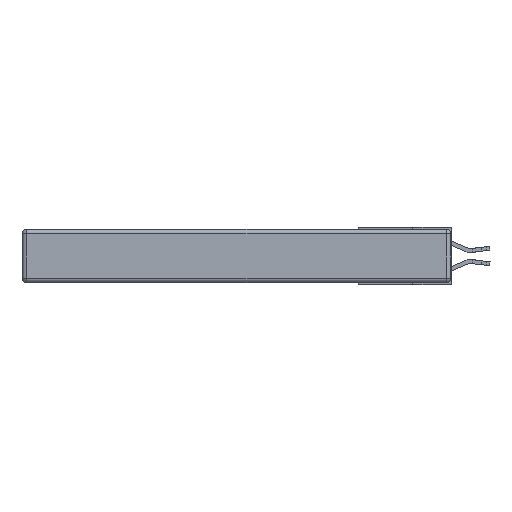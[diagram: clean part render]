
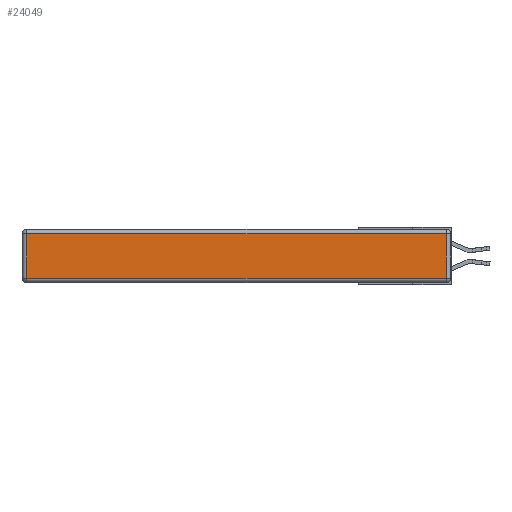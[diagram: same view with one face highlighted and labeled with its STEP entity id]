
A CAD part, left-side view. The second image highlights one B-rep face of the part: STEP entity #24049.
In plain terms, the highlighted planar face has unit normal (-1, 0, 0).
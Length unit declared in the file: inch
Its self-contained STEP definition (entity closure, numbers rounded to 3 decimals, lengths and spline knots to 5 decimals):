
#45 = LINE ( 'NONE', #12397, #9045 ) ;
#1283 = CARTESIAN_POINT ( 'NONE',  ( 0., 0.03, -0.313 ) ) ;
#1310 = DIRECTION ( 'NONE',  ( 0., 0., -1. ) ) ;
#3120 = DIRECTION ( 'NONE',  ( 0., -1., 0. ) ) ;
#3416 = EDGE_CURVE ( 'NONE', #7017, #4889, #10601, .T. ) ;
#4889 = VERTEX_POINT ( 'NONE', #5390 ) ;
#4909 = EDGE_CURVE ( 'NONE', #14106, #7017, #11949, .T. ) ;
#5390 = CARTESIAN_POINT ( 'NONE',  ( 0., 2.72, -0.03 ) ) ;
#5396 = EDGE_CURVE ( 'NONE', #4889, #11838, #45, .T. ) ;
#6542 = CARTESIAN_POINT ( 'NONE',  ( 0., 0., -0.313 ) ) ;
#6829 = CARTESIAN_POINT ( 'NONE',  ( 0., 0.03, -0.03 ) ) ;
#7017 = VERTEX_POINT ( 'NONE', #6829 ) ;
#7033 = CARTESIAN_POINT ( 'NONE',  ( 0., 0.03, -0.343 ) ) ;
#7079 = ORIENTED_EDGE ( 'NONE', *, *, #3416, .T. ) ;
#7637 = PLANE ( 'NONE',  #8991 ) ;
#8047 = ORIENTED_EDGE ( 'NONE', *, *, #17946, .T. ) ;
#8991 = AXIS2_PLACEMENT_3D ( 'NONE', #9500, #22446, #11336 ) ;
#9045 = VECTOR ( 'NONE', #1310, 39.37008 ) ;
#9436 = ORIENTED_EDGE ( 'NONE', *, *, #4909, .T. ) ;
#9500 = CARTESIAN_POINT ( 'NONE',  ( 0., 0., -0.343 ) ) ;
#10601 = LINE ( 'NONE', #21726, #21594 ) ;
#10744 = DIRECTION ( 'NONE',  ( 0., 0., 1. ) ) ;
#11041 = CARTESIAN_POINT ( 'NONE',  ( 0., 2.72, -0.313 ) ) ;
#11336 = DIRECTION ( 'NONE',  ( 0., 0., 1. ) ) ;
#11838 = VERTEX_POINT ( 'NONE', #11041 ) ;
#11949 = LINE ( 'NONE', #7033, #16877 ) ;
#12397 = CARTESIAN_POINT ( 'NONE',  ( 0., 2.72, -0.343 ) ) ;
#12641 = DIRECTION ( 'NONE',  ( 0., 1., 0. ) ) ;
#13711 = EDGE_LOOP ( 'NONE', ( #8047, #9436, #7079, #15920 ) ) ;
#14106 = VERTEX_POINT ( 'NONE', #1283 ) ;
#14936 = VECTOR ( 'NONE', #3120, 39.37008 ) ;
#15920 = ORIENTED_EDGE ( 'NONE', *, *, #5396, .T. ) ;
#16877 = VECTOR ( 'NONE', #10744, 39.37008 ) ;
#17946 = EDGE_CURVE ( 'NONE', #11838, #14106, #23953, .T. ) ;
#21594 = VECTOR ( 'NONE', #12641, 39.37008 ) ;
#21726 = CARTESIAN_POINT ( 'NONE',  ( 0., 2.75, -0.03 ) ) ;
#22402 = FACE_OUTER_BOUND ( 'NONE', #13711, .T. ) ;
#22446 = DIRECTION ( 'NONE',  ( -1., 0., 0. ) ) ;
#23953 = LINE ( 'NONE', #6542, #14936 ) ;
#24049 = ADVANCED_FACE ( 'NONE', ( #22402 ), #7637, .T. ) ;
